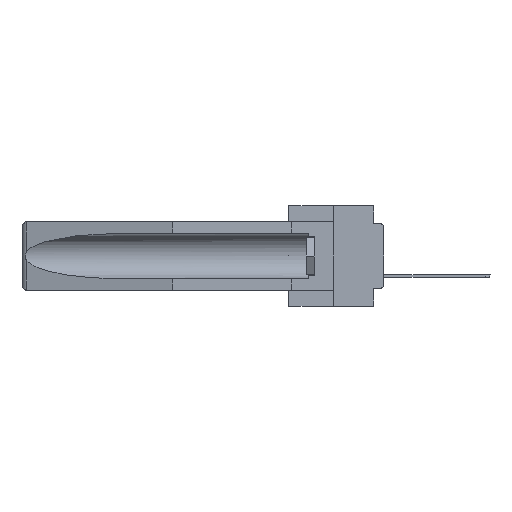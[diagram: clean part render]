
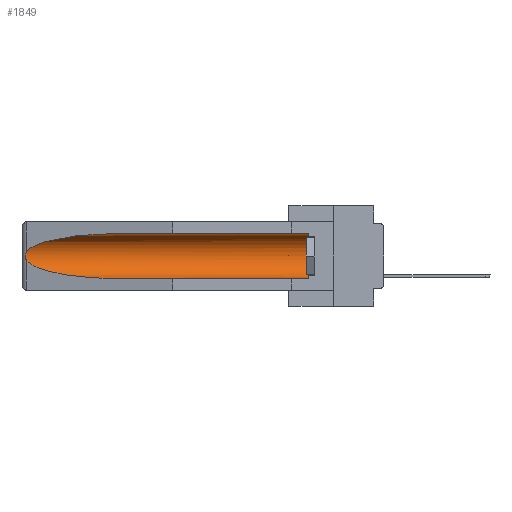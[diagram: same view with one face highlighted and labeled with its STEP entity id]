
A CAD part, left-side view. The second image highlights one B-rep face of the part: STEP entity #1849.
In plain terms, the highlighted cylindrical face has radius 2.857 mm (diameter 5.715 mm), a partial arc.
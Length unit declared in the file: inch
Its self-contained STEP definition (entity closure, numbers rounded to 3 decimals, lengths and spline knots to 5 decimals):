
#1714 =( BOUNDED_CURVE ( )  B_SPLINE_CURVE ( 3, ( #23012, #23761, #2380, #5672 ),
 .UNSPECIFIED., .F., .F. ) 
 B_SPLINE_CURVE_WITH_KNOTS ( ( 4, 4 ),
 ( 0.1948, 1.5708 ),
 .UNSPECIFIED. ) 
 CURVE ( )  GEOMETRIC_REPRESENTATION_ITEM ( )  RATIONAL_B_SPLINE_CURVE ( ( 1., 0.848, 0.848, 1. ) ) 
 REPRESENTATION_ITEM ( '' )  );
#1849 = ADVANCED_FACE ( 'NONE', ( #9428 ), #21301, .F. ) ;
#2380 = CARTESIAN_POINT ( 'NONE',  ( 0.21114, 1.30732, -0.284 ) ) ;
#3779 = ORIENTED_EDGE ( 'NONE', *, *, #27690, .T. ) ;
#4013 = DIRECTION ( 'NONE',  ( 0., -1., 0. ) ) ;
#5672 = CARTESIAN_POINT ( 'NONE',  ( 0.155, 1.07973, -0.284 ) ) ;
#5724 = EDGE_LOOP ( 'NONE', ( #20670, #21070, #30957, #19352, #8748, #3779 ) ) ;
#7467 = VECTOR ( 'NONE', #24727, 39.37008 ) ;
#7557 = VERTEX_POINT ( 'NONE', #19283 ) ;
#7973 = CARTESIAN_POINT ( 'NONE',  ( 0.26597, 1.5296, -0.19026 ) ) ;
#8163 = AXIS2_PLACEMENT_3D ( 'NONE', #19401, #4013, #31260 ) ;
#8164 = CARTESIAN_POINT ( 'NONE',  ( 0.2675, 1.53308, -0.17534 ) ) ;
#8748 = ORIENTED_EDGE ( 'NONE', *, *, #31526, .T. ) ;
#9239 = DIRECTION ( 'NONE',  ( 0., 1., 0. ) ) ;
#9428 = FACE_OUTER_BOUND ( 'NONE', #5724, .T. ) ;
#12047 = CARTESIAN_POINT ( 'NONE',  ( 0.26537, 1.52718, -0.19328 ) ) ;
#12163 =( BOUNDED_CURVE ( )  B_SPLINE_CURVE ( 3, ( #38192, #35471, #17617, #29456 ),
 .UNSPECIFIED., .F., .F. ) 
 B_SPLINE_CURVE_WITH_KNOTS ( ( 4, 4 ),
 ( 4.71239, 6.08839 ),
 .UNSPECIFIED. ) 
 CURVE ( )  GEOMETRIC_REPRESENTATION_ITEM ( )  RATIONAL_B_SPLINE_CURVE ( ( 1., 0.848, 0.848, 1. ) ) 
 REPRESENTATION_ITEM ( '' )  );
#13170 = CARTESIAN_POINT ( 'NONE',  ( 0.155, -0.30754, -0.059 ) ) ;
#13190 = CARTESIAN_POINT ( 'NONE',  ( 0.155, 1.07973, -0.059 ) ) ;
#14009 = CARTESIAN_POINT ( 'NONE',  ( 0.2673, 1.53269, -0.17917 ) ) ;
#15099 = CARTESIAN_POINT ( 'NONE',  ( 0.155, 0.126, -0.284 ) ) ;
#15728 = LINE ( 'NONE', #13170, #22508 ) ;
#17372 = AXIS2_PLACEMENT_3D ( 'NONE', #29857, #9239, #33153 ) ;
#17617 = CARTESIAN_POINT ( 'NONE',  ( 0.25451, 1.48313, -0.09465 ) ) ;
#18898 = LINE ( 'NONE', #31342, #7467 ) ;
#19283 = CARTESIAN_POINT ( 'NONE',  ( 0.26537, 1.52718, -0.14972 ) ) ;
#19352 = ORIENTED_EDGE ( 'NONE', *, *, #25441, .F. ) ;
#19401 = CARTESIAN_POINT ( 'NONE',  ( 0.155, 0.126, -0.1715 ) ) ;
#20026 = CARTESIAN_POINT ( 'NONE',  ( 0.26655, 1.53094, -0.18657 ) ) ;
#20670 = ORIENTED_EDGE ( 'NONE', *, *, #24695, .T. ) ;
#21070 = ORIENTED_EDGE ( 'NONE', *, *, #33624, .T. ) ;
#21301 = CYLINDRICAL_SURFACE ( 'NONE', #17372, 0.1125 ) ;
#22508 = VECTOR ( 'NONE', #24646, 39.37008 ) ;
#22565 = CARTESIAN_POINT ( 'NONE',  ( 0.26537, 1.52718, -0.14972 ) ) ;
#22754 = CARTESIAN_POINT ( 'NONE',  ( 0.2675, 1.53308, -0.16763 ) ) ;
#23012 = CARTESIAN_POINT ( 'NONE',  ( 0.26537, 1.52718, -0.19328 ) ) ;
#23154 = VERTEX_POINT ( 'NONE', #12047 ) ;
#23761 = CARTESIAN_POINT ( 'NONE',  ( 0.25451, 1.48313, -0.24835 ) ) ;
#24646 = DIRECTION ( 'NONE',  ( 0., 1., 0. ) ) ;
#24695 = EDGE_CURVE ( 'NONE', #33893, #7557, #12163, .T. ) ;
#24727 = DIRECTION ( 'NONE',  ( 0., 1., 0. ) ) ;
#25441 = EDGE_CURVE ( 'NONE', #31826, #26435, #18898, .T. ) ;
#25492 = B_SPLINE_CURVE_WITH_KNOTS ( 'NONE', 3,
 ( #22565, #34237, #34802, #28205, #22754, #8164, #14009, #20026, #7973, #37122 ),
 .UNSPECIFIED., .F., .F.,
 ( 4, 2, 2, 2, 4 ),
 ( 0., 0.00029, 0.00058, 0.00087, 0.00117 ),
 .UNSPECIFIED. ) ;
#26140 = VERTEX_POINT ( 'NONE', #30447 ) ;
#26435 = VERTEX_POINT ( 'NONE', #29610 ) ;
#27690 = EDGE_CURVE ( 'NONE', #26140, #33893, #15728, .T. ) ;
#28205 = CARTESIAN_POINT ( 'NONE',  ( 0.2673, 1.5327, -0.16383 ) ) ;
#29165 = EDGE_CURVE ( 'NONE', #23154, #26435, #1714, .T. ) ;
#29456 = CARTESIAN_POINT ( 'NONE',  ( 0.26537, 1.52718, -0.14972 ) ) ;
#29610 = CARTESIAN_POINT ( 'NONE',  ( 0.155, 1.07973, -0.284 ) ) ;
#29857 = CARTESIAN_POINT ( 'NONE',  ( 0.155, -0.30754, -0.1715 ) ) ;
#30447 = CARTESIAN_POINT ( 'NONE',  ( 0.155, 0.126, -0.059 ) ) ;
#30957 = ORIENTED_EDGE ( 'NONE', *, *, #29165, .T. ) ;
#31260 = DIRECTION ( 'NONE',  ( 0., 0., 1. ) ) ;
#31342 = CARTESIAN_POINT ( 'NONE',  ( 0.155, -0.30754, -0.284 ) ) ;
#31526 = EDGE_CURVE ( 'NONE', #31826, #26140, #33614, .T. ) ;
#31826 = VERTEX_POINT ( 'NONE', #15099 ) ;
#33153 = DIRECTION ( 'NONE',  ( 0., 0., 1. ) ) ;
#33614 = CIRCLE ( 'NONE', #8163, 0.1125 ) ;
#33624 = EDGE_CURVE ( 'NONE', #7557, #23154, #25492, .T. ) ;
#33893 = VERTEX_POINT ( 'NONE', #13190 ) ;
#34237 = CARTESIAN_POINT ( 'NONE',  ( 0.26597, 1.52961, -0.15275 ) ) ;
#34802 = CARTESIAN_POINT ( 'NONE',  ( 0.26654, 1.53092, -0.15636 ) ) ;
#35471 = CARTESIAN_POINT ( 'NONE',  ( 0.21114, 1.30732, -0.059 ) ) ;
#37122 = CARTESIAN_POINT ( 'NONE',  ( 0.26537, 1.52718, -0.19328 ) ) ;
#38192 = CARTESIAN_POINT ( 'NONE',  ( 0.155, 1.07973, -0.059 ) ) ;
